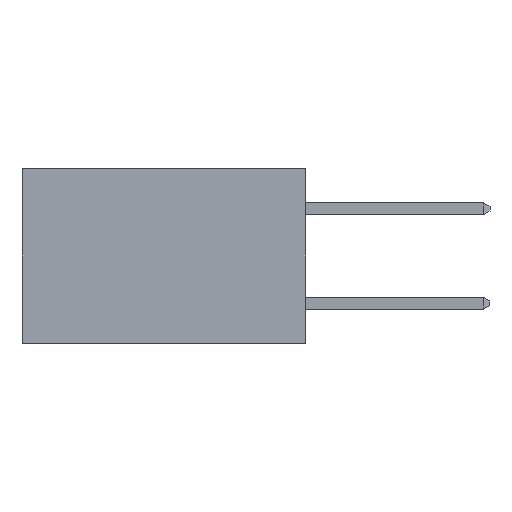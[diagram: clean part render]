
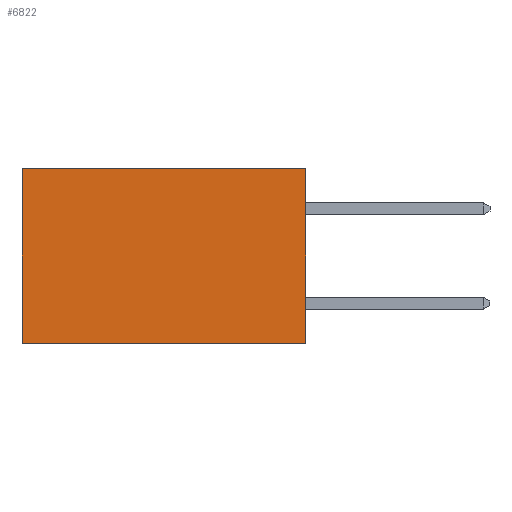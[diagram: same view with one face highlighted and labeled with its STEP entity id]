
A CAD part, left-side view. The second image highlights one B-rep face of the part: STEP entity #6822.
In plain terms, the highlighted planar face has unit normal (-1, 0, 0).
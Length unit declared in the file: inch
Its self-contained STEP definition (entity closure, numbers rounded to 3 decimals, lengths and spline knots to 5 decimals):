
#117 = VERTEX_POINT ( 'NONE', #1829 ) ;
#343 = ORIENTED_EDGE ( 'NONE', *, *, #4697, .T. ) ;
#560 = CARTESIAN_POINT ( 'NONE',  ( 0.298, 0., -0.37 ) ) ;
#638 = VERTEX_POINT ( 'NONE', #7143 ) ;
#798 = LINE ( 'NONE', #5328, #8584 ) ;
#1322 = EDGE_CURVE ( 'NONE', #8286, #638, #7269, .T. ) ;
#1690 = DIRECTION ( 'NONE',  ( 0., 0., -1. ) ) ;
#1709 = CARTESIAN_POINT ( 'NONE',  ( 0.298, 0.6, 0. ) ) ;
#1725 = CARTESIAN_POINT ( 'NONE',  ( 0.298, 0., 0. ) ) ;
#1829 = CARTESIAN_POINT ( 'NONE',  ( 0.298, 0.6, 0. ) ) ;
#2190 = ORIENTED_EDGE ( 'NONE', *, *, #1322, .F. ) ;
#2267 = LINE ( 'NONE', #1709, #2746 ) ;
#2334 = EDGE_CURVE ( 'NONE', #117, #638, #2267, .T. ) ;
#2746 = VECTOR ( 'NONE', #1690, 39.37008 ) ;
#4202 = ORIENTED_EDGE ( 'NONE', *, *, #7349, .F. ) ;
#4348 = VECTOR ( 'NONE', #6330, 39.37008 ) ;
#4603 = DIRECTION ( 'NONE',  ( 0., 1., 0. ) ) ;
#4697 = EDGE_CURVE ( 'NONE', #7965, #117, #798, .T. ) ;
#4843 = FACE_OUTER_BOUND ( 'NONE', #8206, .T. ) ;
#5265 = VECTOR ( 'NONE', #4603, 39.37008 ) ;
#5328 = CARTESIAN_POINT ( 'NONE',  ( 0.298, 0., 0. ) ) ;
#5925 = DIRECTION ( 'NONE',  ( 1., 0., 0. ) ) ;
#6027 = DIRECTION ( 'NONE',  ( 0., 0., -1. ) ) ;
#6146 = CARTESIAN_POINT ( 'NONE',  ( 0.298, 0., 0. ) ) ;
#6330 = DIRECTION ( 'NONE',  ( 0., 0., -1. ) ) ;
#6372 = LINE ( 'NONE', #6443, #4348 ) ;
#6443 = CARTESIAN_POINT ( 'NONE',  ( 0.298, 0., 0. ) ) ;
#6723 = AXIS2_PLACEMENT_3D ( 'NONE', #6146, #5925, #6027 ) ;
#6822 = ADVANCED_FACE ( 'NONE', ( #4843 ), #6886, .F. ) ;
#6886 = PLANE ( 'NONE',  #6723 ) ;
#7143 = CARTESIAN_POINT ( 'NONE',  ( 0.298, 0.6, -0.37 ) ) ;
#7269 = LINE ( 'NONE', #8641, #5265 ) ;
#7349 = EDGE_CURVE ( 'NONE', #7965, #8286, #6372, .T. ) ;
#7965 = VERTEX_POINT ( 'NONE', #1725 ) ;
#7987 = ORIENTED_EDGE ( 'NONE', *, *, #2334, .T. ) ;
#8206 = EDGE_LOOP ( 'NONE', ( #7987, #2190, #4202, #343 ) ) ;
#8286 = VERTEX_POINT ( 'NONE', #560 ) ;
#8541 = DIRECTION ( 'NONE',  ( 0., 1., 0. ) ) ;
#8584 = VECTOR ( 'NONE', #8541, 39.37008 ) ;
#8641 = CARTESIAN_POINT ( 'NONE',  ( 0.298, 0., -0.37 ) ) ;
